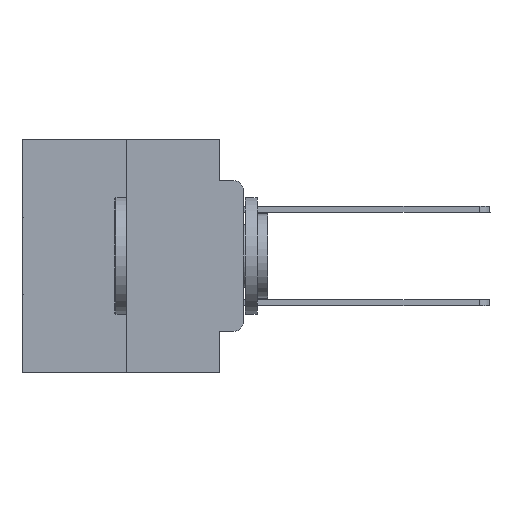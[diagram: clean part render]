
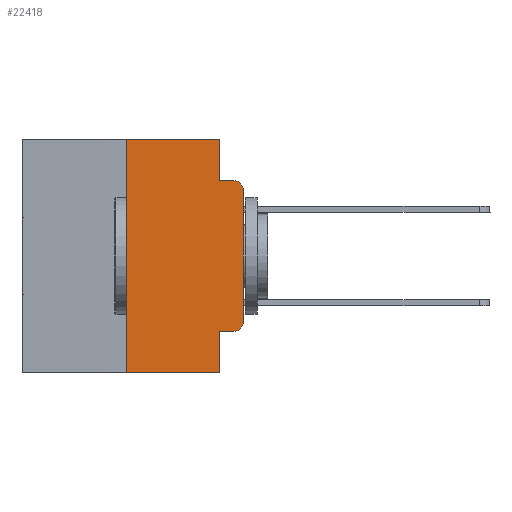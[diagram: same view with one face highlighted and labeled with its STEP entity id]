
A CAD part, left-side view. The second image highlights one B-rep face of the part: STEP entity #22418.
In plain terms, the highlighted planar face has unit normal (-1, 0, 0).
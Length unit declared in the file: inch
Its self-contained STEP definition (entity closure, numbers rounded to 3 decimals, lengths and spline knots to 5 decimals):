
#222 = DIRECTION ( 'NONE',  ( -1., 0., 0. ) ) ;
#261 = VERTEX_POINT ( 'NONE', #20542 ) ;
#353 = ORIENTED_EDGE ( 'NONE', *, *, #7492, .F. ) ;
#1131 = CARTESIAN_POINT ( 'NONE',  ( 0., 0.051, -0.0885 ) ) ;
#1411 = DIRECTION ( 'NONE',  ( 0., -1., 0. ) ) ;
#1559 = VERTEX_POINT ( 'NONE', #12263 ) ;
#2644 = LINE ( 'NONE', #28119, #3694 ) ;
#3694 = VECTOR ( 'NONE', #21097, 39.37008 ) ;
#3828 = VECTOR ( 'NONE', #1411, 39.37008 ) ;
#4104 = FACE_OUTER_BOUND ( 'NONE', #24491, .T. ) ;
#4135 = EDGE_CURVE ( 'NONE', #6407, #24692, #12161, .T. ) ;
#4463 = VECTOR ( 'NONE', #19300, 39.37008 ) ;
#5050 = AXIS2_PLACEMENT_3D ( 'NONE', #13635, #222, #23488 ) ;
#5373 = CARTESIAN_POINT ( 'NONE',  ( 0., 0.25, 0. ) ) ;
#5376 = EDGE_CURVE ( 'NONE', #27861, #23504, #15691, .T. ) ;
#5511 = EDGE_CURVE ( 'NONE', #18233, #13887, #2644, .T. ) ;
#5552 = AXIS2_PLACEMENT_3D ( 'NONE', #29041, #22757, #27126 ) ;
#6187 = EDGE_CURVE ( 'NONE', #27861, #261, #21968, .T. ) ;
#6318 = VECTOR ( 'NONE', #29262, 39.37008 ) ;
#6352 = VERTEX_POINT ( 'NONE', #28799 ) ;
#6407 = VERTEX_POINT ( 'NONE', #11793 ) ;
#6488 = CIRCLE ( 'NONE', #20875, 0.02 ) ;
#6525 = CARTESIAN_POINT ( 'NONE',  ( 0., 0.473, 0. ) ) ;
#6536 = EDGE_CURVE ( 'NONE', #18233, #261, #7066, .T. ) ;
#7037 = LINE ( 'NONE', #24107, #6318 ) ;
#7066 = LINE ( 'NONE', #22372, #3828 ) ;
#7492 = EDGE_CURVE ( 'NONE', #21818, #6352, #7037, .T. ) ;
#8546 = LINE ( 'NONE', #12345, #24849 ) ;
#9019 = VECTOR ( 'NONE', #20516, 39.37008 ) ;
#9990 = DIRECTION ( 'NONE',  ( 0., 0., 1. ) ) ;
#10698 = EDGE_CURVE ( 'NONE', #24692, #6352, #6488, .T. ) ;
#11793 = CARTESIAN_POINT ( 'NONE',  ( 0., 0., -0.3915 ) ) ;
#12022 = ORIENTED_EDGE ( 'NONE', *, *, #5511, .F. ) ;
#12161 = LINE ( 'NONE', #16912, #21225 ) ;
#12263 = CARTESIAN_POINT ( 'NONE',  ( 0., 0.051, 0. ) ) ;
#12345 = CARTESIAN_POINT ( 'NONE',  ( 0., 0.051, 0. ) ) ;
#12804 = ORIENTED_EDGE ( 'NONE', *, *, #10698, .T. ) ;
#13635 = CARTESIAN_POINT ( 'NONE',  ( 0., 0.02, -0.3915 ) ) ;
#13887 = VERTEX_POINT ( 'NONE', #5373 ) ;
#13979 = VECTOR ( 'NONE', #18826, 39.37008 ) ;
#14439 = DIRECTION ( 'NONE',  ( 0., 0., -1. ) ) ;
#14458 = EDGE_CURVE ( 'NONE', #23504, #6407, #19596, .T. ) ;
#14968 = DIRECTION ( 'NONE',  ( 0., 0., -1. ) ) ;
#15151 = CARTESIAN_POINT ( 'NONE',  ( 0., 0.051, -0.4115 ) ) ;
#15691 = LINE ( 'NONE', #24273, #4463 ) ;
#15785 = EDGE_CURVE ( 'NONE', #13887, #1559, #26822, .T. ) ;
#16912 = CARTESIAN_POINT ( 'NONE',  ( 0., 0., 0. ) ) ;
#17425 = ORIENTED_EDGE ( 'NONE', *, *, #6187, .F. ) ;
#17830 = ORIENTED_EDGE ( 'NONE', *, *, #14458, .T. ) ;
#18233 = VERTEX_POINT ( 'NONE', #24904 ) ;
#18431 = ORIENTED_EDGE ( 'NONE', *, *, #6536, .T. ) ;
#18826 = DIRECTION ( 'NONE',  ( 0., 0., -1. ) ) ;
#19300 = DIRECTION ( 'NONE',  ( 0., -1., 0. ) ) ;
#19596 = CIRCLE ( 'NONE', #5050, 0.02 ) ;
#19706 = PLANE ( 'NONE',  #5552 ) ;
#20516 = DIRECTION ( 'NONE',  ( 0., -1., 0. ) ) ;
#20542 = CARTESIAN_POINT ( 'NONE',  ( 0., 0.051, -0.5 ) ) ;
#20546 = ORIENTED_EDGE ( 'NONE', *, *, #5376, .T. ) ;
#20875 = AXIS2_PLACEMENT_3D ( 'NONE', #21341, #28374, #14439 ) ;
#21097 = DIRECTION ( 'NONE',  ( 0., 0., 1. ) ) ;
#21225 = VECTOR ( 'NONE', #9990, 39.37008 ) ;
#21341 = CARTESIAN_POINT ( 'NONE',  ( 0., 0.02, -0.1085 ) ) ;
#21818 = VERTEX_POINT ( 'NONE', #1131 ) ;
#21968 = LINE ( 'NONE', #25945, #13979 ) ;
#22372 = CARTESIAN_POINT ( 'NONE',  ( 0., 0.473, -0.5 ) ) ;
#22418 = ADVANCED_FACE ( 'NONE', ( #4104 ), #19706, .F. ) ;
#22725 = ORIENTED_EDGE ( 'NONE', *, *, #4135, .T. ) ;
#22757 = DIRECTION ( 'NONE',  ( 1., 0., 0. ) ) ;
#23488 = DIRECTION ( 'NONE',  ( 0., 0., -1. ) ) ;
#23504 = VERTEX_POINT ( 'NONE', #28502 ) ;
#24107 = CARTESIAN_POINT ( 'NONE',  ( 0., 0.051, -0.0885 ) ) ;
#24273 = CARTESIAN_POINT ( 'NONE',  ( 0., 0.051, -0.4115 ) ) ;
#24491 = EDGE_LOOP ( 'NONE', ( #22725, #12804, #353, #25220, #27516, #12022, #18431, #17425, #20546, #17830 ) ) ;
#24692 = VERTEX_POINT ( 'NONE', #27217 ) ;
#24849 = VECTOR ( 'NONE', #14968, 39.37008 ) ;
#24904 = CARTESIAN_POINT ( 'NONE',  ( 0., 0.25, -0.5 ) ) ;
#25220 = ORIENTED_EDGE ( 'NONE', *, *, #25751, .F. ) ;
#25751 = EDGE_CURVE ( 'NONE', #1559, #21818, #8546, .T. ) ;
#25945 = CARTESIAN_POINT ( 'NONE',  ( 0., 0.051, 0. ) ) ;
#26822 = LINE ( 'NONE', #6525, #9019 ) ;
#27126 = DIRECTION ( 'NONE',  ( 0., 0., -1. ) ) ;
#27217 = CARTESIAN_POINT ( 'NONE',  ( 0., 0., -0.1085 ) ) ;
#27516 = ORIENTED_EDGE ( 'NONE', *, *, #15785, .F. ) ;
#27861 = VERTEX_POINT ( 'NONE', #15151 ) ;
#28119 = CARTESIAN_POINT ( 'NONE',  ( 0., 0.25, 0. ) ) ;
#28374 = DIRECTION ( 'NONE',  ( -1., 0., 0. ) ) ;
#28502 = CARTESIAN_POINT ( 'NONE',  ( 0., 0.02, -0.4115 ) ) ;
#28799 = CARTESIAN_POINT ( 'NONE',  ( 0., 0.02, -0.0885 ) ) ;
#29041 = CARTESIAN_POINT ( 'NONE',  ( 0., 0.473, 0. ) ) ;
#29262 = DIRECTION ( 'NONE',  ( 0., -1., 0. ) ) ;
